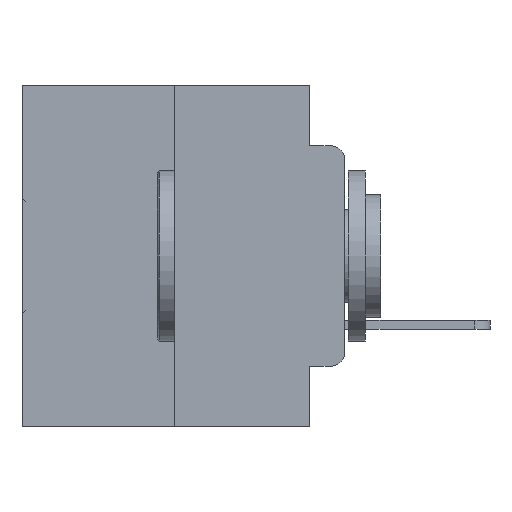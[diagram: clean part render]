
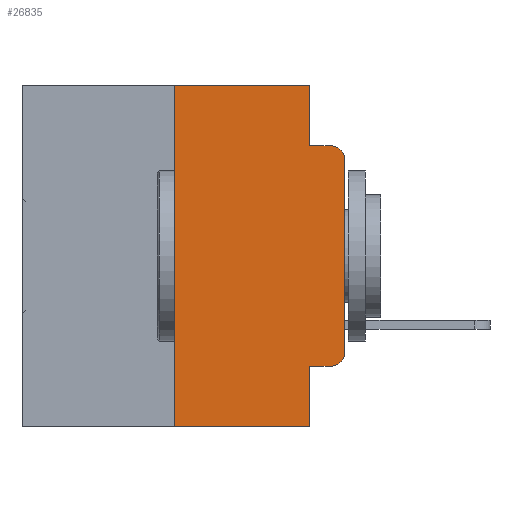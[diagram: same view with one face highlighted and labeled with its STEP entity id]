
A CAD part, left-side view. The second image highlights one B-rep face of the part: STEP entity #26835.
In plain terms, the highlighted planar face has unit normal (-1, 0, 0).
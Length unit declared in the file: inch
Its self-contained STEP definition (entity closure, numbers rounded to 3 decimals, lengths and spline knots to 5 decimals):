
#374 = CARTESIAN_POINT ( 'NONE',  ( 0., 0.051, -0.0885 ) ) ;
#683 = VECTOR ( 'NONE', #26455, 39.37008 ) ;
#867 = LINE ( 'NONE', #1680, #20878 ) ;
#1680 = CARTESIAN_POINT ( 'NONE',  ( 0., 0.051, 0. ) ) ;
#2245 = VERTEX_POINT ( 'NONE', #374 ) ;
#2397 = VERTEX_POINT ( 'NONE', #9921 ) ;
#3486 = LINE ( 'NONE', #29244, #23207 ) ;
#4223 = CARTESIAN_POINT ( 'NONE',  ( 0., 0.051, -0.0885 ) ) ;
#4236 = AXIS2_PLACEMENT_3D ( 'NONE', #27050, #12195, #29348 ) ;
#4717 = VECTOR ( 'NONE', #17792, 39.37008 ) ;
#5096 = VERTEX_POINT ( 'NONE', #8917 ) ;
#5428 = DIRECTION ( 'NONE',  ( -1., 0., 0. ) ) ;
#6101 = CARTESIAN_POINT ( 'NONE',  ( 0., 0.02, -0.0885 ) ) ;
#7827 = CIRCLE ( 'NONE', #21521, 0.02 ) ;
#7875 = CARTESIAN_POINT ( 'NONE',  ( 0., 0., -0.3915 ) ) ;
#8184 = VERTEX_POINT ( 'NONE', #7875 ) ;
#8917 = CARTESIAN_POINT ( 'NONE',  ( 0., 0.051, -0.4115 ) ) ;
#9055 = CARTESIAN_POINT ( 'NONE',  ( 0., 0.473, 0. ) ) ;
#9076 = VECTOR ( 'NONE', #17176, 39.37008 ) ;
#9463 = VERTEX_POINT ( 'NONE', #25468 ) ;
#9573 = PLANE ( 'NONE',  #10173 ) ;
#9907 = DIRECTION ( 'NONE',  ( 0., 0., -1. ) ) ;
#9921 = CARTESIAN_POINT ( 'NONE',  ( 0., 0.02, -0.4115 ) ) ;
#10173 = AXIS2_PLACEMENT_3D ( 'NONE', #24574, #12072, #29219 ) ;
#10222 = CARTESIAN_POINT ( 'NONE',  ( 0., 0.051, 0. ) ) ;
#10434 = VERTEX_POINT ( 'NONE', #6101 ) ;
#10494 = EDGE_CURVE ( 'NONE', #17200, #16877, #16375, .T. ) ;
#10515 = ORIENTED_EDGE ( 'NONE', *, *, #13783, .T. ) ;
#10882 = ORIENTED_EDGE ( 'NONE', *, *, #13786, .T. ) ;
#11494 = ORIENTED_EDGE ( 'NONE', *, *, #13788, .F. ) ;
#11758 = ORIENTED_EDGE ( 'NONE', *, *, #13838, .F. ) ;
#11780 = LINE ( 'NONE', #15282, #4717 ) ;
#12072 = DIRECTION ( 'NONE',  ( 1., 0., 0. ) ) ;
#12095 = DIRECTION ( 'NONE',  ( 0., 0., 1. ) ) ;
#12195 = DIRECTION ( 'NONE',  ( -1., 0., 0. ) ) ;
#12242 = ORIENTED_EDGE ( 'NONE', *, *, #10494, .F. ) ;
#12836 = ORIENTED_EDGE ( 'NONE', *, *, #13932, .F. ) ;
#12888 = EDGE_CURVE ( 'NONE', #14807, #9463, #24800, .T. ) ;
#12955 = ORIENTED_EDGE ( 'NONE', *, *, #12888, .T. ) ;
#13352 = ORIENTED_EDGE ( 'NONE', *, *, #13936, .F. ) ;
#13649 = ORIENTED_EDGE ( 'NONE', *, *, #14033, .T. ) ;
#13783 = EDGE_CURVE ( 'NONE', #8184, #29910, #3486, .T. ) ;
#13786 = EDGE_CURVE ( 'NONE', #29910, #10434, #28731, .T. ) ;
#13788 = EDGE_CURVE ( 'NONE', #2245, #10434, #22438, .T. ) ;
#13838 = EDGE_CURVE ( 'NONE', #16877, #2245, #867, .T. ) ;
#13932 = EDGE_CURVE ( 'NONE', #14807, #17200, #11780, .T. ) ;
#13936 = EDGE_CURVE ( 'NONE', #5096, #9463, #18473, .T. ) ;
#13941 = CARTESIAN_POINT ( 'NONE',  ( 0., 0.051, 0. ) ) ;
#13979 = ORIENTED_EDGE ( 'NONE', *, *, #14036, .T. ) ;
#14033 = EDGE_CURVE ( 'NONE', #5096, #2397, #27632, .T. ) ;
#14036 = EDGE_CURVE ( 'NONE', #2397, #8184, #7827, .T. ) ;
#14322 = FACE_OUTER_BOUND ( 'NONE', #27601, .T. ) ;
#14807 = VERTEX_POINT ( 'NONE', #31158 ) ;
#15282 = CARTESIAN_POINT ( 'NONE',  ( 0., 0.25, 0. ) ) ;
#16375 = LINE ( 'NONE', #9055, #683 ) ;
#16877 = VERTEX_POINT ( 'NONE', #13941 ) ;
#17176 = DIRECTION ( 'NONE',  ( 0., -1., 0. ) ) ;
#17200 = VERTEX_POINT ( 'NONE', #27899 ) ;
#17792 = DIRECTION ( 'NONE',  ( 0., 0., 1. ) ) ;
#18473 = LINE ( 'NONE', #10222, #25095 ) ;
#20259 = DIRECTION ( 'NONE',  ( 0., 0., -1. ) ) ;
#20800 = CARTESIAN_POINT ( 'NONE',  ( 0., 0.02, -0.3915 ) ) ;
#20878 = VECTOR ( 'NONE', #9907, 39.37008 ) ;
#21521 = AXIS2_PLACEMENT_3D ( 'NONE', #20800, #5428, #23298 ) ;
#22038 = VECTOR ( 'NONE', #30218, 39.37008 ) ;
#22438 = LINE ( 'NONE', #4223, #9076 ) ;
#23207 = VECTOR ( 'NONE', #12095, 39.37008 ) ;
#23298 = DIRECTION ( 'NONE',  ( 0., 0., -1. ) ) ;
#24574 = CARTESIAN_POINT ( 'NONE',  ( 0., 0.473, 0. ) ) ;
#24793 = CARTESIAN_POINT ( 'NONE',  ( 0., 0., -0.1085 ) ) ;
#24800 = LINE ( 'NONE', #26179, #30202 ) ;
#25095 = VECTOR ( 'NONE', #20259, 39.37008 ) ;
#25468 = CARTESIAN_POINT ( 'NONE',  ( 0., 0.051, -0.5 ) ) ;
#26179 = CARTESIAN_POINT ( 'NONE',  ( 0., 0.473, -0.5 ) ) ;
#26455 = DIRECTION ( 'NONE',  ( 0., -1., 0. ) ) ;
#26835 = ADVANCED_FACE ( 'NONE', ( #14322 ), #9573, .F. ) ;
#27050 = CARTESIAN_POINT ( 'NONE',  ( 0., 0.02, -0.1085 ) ) ;
#27601 = EDGE_LOOP ( 'NONE', ( #10515, #10882, #11494, #11758, #12242, #12836, #12955, #13352, #13649, #13979 ) ) ;
#27632 = LINE ( 'NONE', #27935, #22038 ) ;
#27899 = CARTESIAN_POINT ( 'NONE',  ( 0., 0.25, 0. ) ) ;
#27935 = CARTESIAN_POINT ( 'NONE',  ( 0., 0.051, -0.4115 ) ) ;
#28499 = DIRECTION ( 'NONE',  ( 0., -1., 0. ) ) ;
#28731 = CIRCLE ( 'NONE', #4236, 0.02 ) ;
#29219 = DIRECTION ( 'NONE',  ( 0., 0., -1. ) ) ;
#29244 = CARTESIAN_POINT ( 'NONE',  ( 0., 0., 0. ) ) ;
#29348 = DIRECTION ( 'NONE',  ( 0., 0., -1. ) ) ;
#29910 = VERTEX_POINT ( 'NONE', #24793 ) ;
#30202 = VECTOR ( 'NONE', #28499, 39.37008 ) ;
#30218 = DIRECTION ( 'NONE',  ( 0., -1., 0. ) ) ;
#31158 = CARTESIAN_POINT ( 'NONE',  ( 0., 0.25, -0.5 ) ) ;
